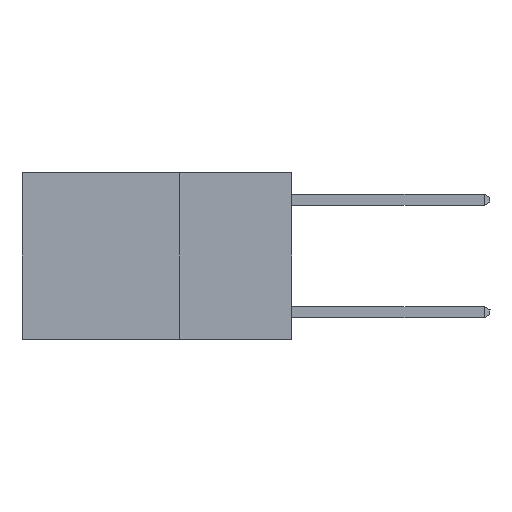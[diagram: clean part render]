
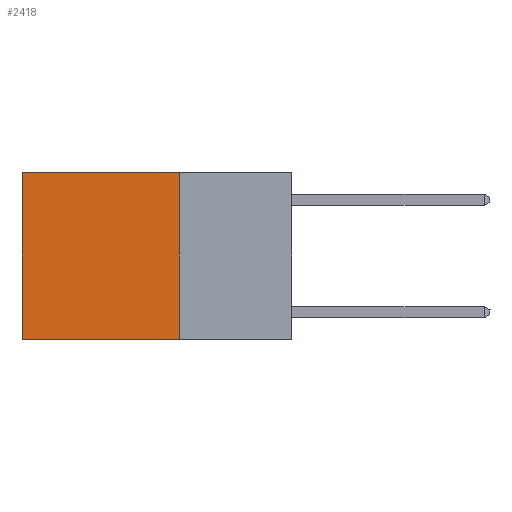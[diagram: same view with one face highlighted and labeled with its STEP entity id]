
A CAD part, left-side view. The second image highlights one B-rep face of the part: STEP entity #2418.
In plain terms, the highlighted planar face has unit normal (-1, 0, 0).
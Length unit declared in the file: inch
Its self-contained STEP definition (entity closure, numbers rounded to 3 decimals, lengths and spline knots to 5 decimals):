
#990 = EDGE_CURVE ( 'NONE', #13094, #5028, #10035, .T. ) ;
#1032 = CARTESIAN_POINT ( 'NONE',  ( 0.2625, 0.25, 0. ) ) ;
#2418 = ADVANCED_FACE ( 'NONE', ( #3967 ), #9922, .F. ) ;
#2542 = DIRECTION ( 'NONE',  ( 0., 0., -1. ) ) ;
#2679 = VECTOR ( 'NONE', #15101, 39.37008 ) ;
#3150 = LINE ( 'NONE', #10712, #2679 ) ;
#3967 = FACE_OUTER_BOUND ( 'NONE', #10839, .T. ) ;
#4029 = CARTESIAN_POINT ( 'NONE',  ( 0.2625, 0.25, 0. ) ) ;
#4262 = VECTOR ( 'NONE', #17214, 39.37008 ) ;
#5028 = VERTEX_POINT ( 'NONE', #14113 ) ;
#5566 = LINE ( 'NONE', #12845, #12888 ) ;
#6777 = EDGE_CURVE ( 'NONE', #13094, #13604, #8215, .T. ) ;
#7928 = CARTESIAN_POINT ( 'NONE',  ( 0.2625, 0.6, 0. ) ) ;
#8091 = ORIENTED_EDGE ( 'NONE', *, *, #18228, .F. ) ;
#8215 = LINE ( 'NONE', #4029, #4262 ) ;
#8456 = CARTESIAN_POINT ( 'NONE',  ( 0.2625, 0.25, 0. ) ) ;
#9914 = DIRECTION ( 'NONE',  ( 0., 1., 0. ) ) ;
#9922 = PLANE ( 'NONE',  #15857 ) ;
#10035 = LINE ( 'NONE', #16954, #12994 ) ;
#10247 = ORIENTED_EDGE ( 'NONE', *, *, #990, .F. ) ;
#10712 = CARTESIAN_POINT ( 'NONE',  ( 0.2625, 0.6, 0. ) ) ;
#10839 = EDGE_LOOP ( 'NONE', ( #16918, #8091, #10247, #12790 ) ) ;
#11398 = DIRECTION ( 'NONE',  ( 1., 0., 0. ) ) ;
#12790 = ORIENTED_EDGE ( 'NONE', *, *, #6777, .T. ) ;
#12845 = CARTESIAN_POINT ( 'NONE',  ( 0.2625, 0.25, -0.37 ) ) ;
#12888 = VECTOR ( 'NONE', #9914, 39.37008 ) ;
#12994 = VECTOR ( 'NONE', #17009, 39.37008 ) ;
#13094 = VERTEX_POINT ( 'NONE', #1032 ) ;
#13604 = VERTEX_POINT ( 'NONE', #7928 ) ;
#13750 = CARTESIAN_POINT ( 'NONE',  ( 0.2625, 0.6, -0.37 ) ) ;
#14080 = EDGE_CURVE ( 'NONE', #13604, #15837, #3150, .T. ) ;
#14113 = CARTESIAN_POINT ( 'NONE',  ( 0.2625, 0.25, -0.37 ) ) ;
#15101 = DIRECTION ( 'NONE',  ( 0., 0., -1. ) ) ;
#15837 = VERTEX_POINT ( 'NONE', #13750 ) ;
#15857 = AXIS2_PLACEMENT_3D ( 'NONE', #8456, #11398, #2542 ) ;
#16918 = ORIENTED_EDGE ( 'NONE', *, *, #14080, .T. ) ;
#16954 = CARTESIAN_POINT ( 'NONE',  ( 0.2625, 0.25, 0. ) ) ;
#17009 = DIRECTION ( 'NONE',  ( 0., 0., -1. ) ) ;
#17214 = DIRECTION ( 'NONE',  ( 0., 1., 0. ) ) ;
#18228 = EDGE_CURVE ( 'NONE', #5028, #15837, #5566, .T. ) ;
